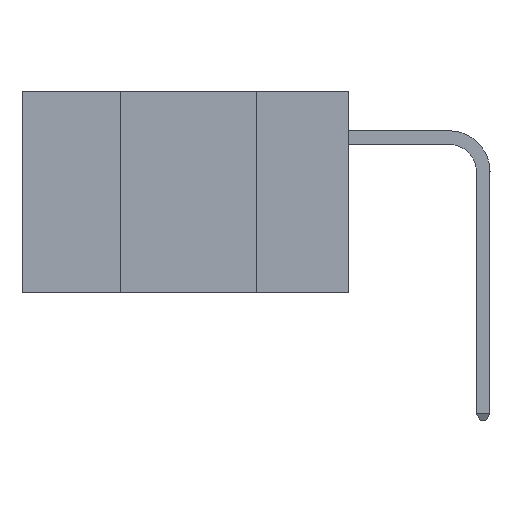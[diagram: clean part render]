
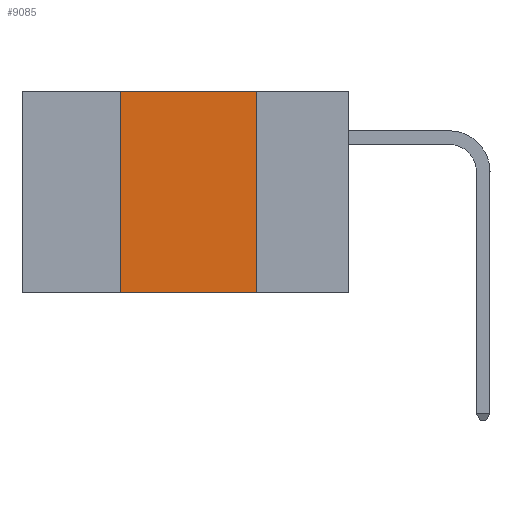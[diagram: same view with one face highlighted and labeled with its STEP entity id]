
A CAD part, left-side view. The second image highlights one B-rep face of the part: STEP entity #9085.
In plain terms, the highlighted planar face has unit normal (-1, 0, 0).
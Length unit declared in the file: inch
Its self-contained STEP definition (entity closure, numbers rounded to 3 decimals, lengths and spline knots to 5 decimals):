
#178 = EDGE_LOOP ( 'NONE', ( #279, #3613, #8611, #1136 ) ) ;
#191 = VERTEX_POINT ( 'NONE', #4057 ) ;
#196 = VERTEX_POINT ( 'NONE', #4852 ) ;
#248 = DIRECTION ( 'NONE',  ( 1., 0., 0. ) ) ;
#279 = ORIENTED_EDGE ( 'NONE', *, *, #11119, .F. ) ;
#324 = DIRECTION ( 'NONE',  ( 0., 0., -1. ) ) ;
#400 = VECTOR ( 'NONE', #6209, 39.37008 ) ;
#1136 = ORIENTED_EDGE ( 'NONE', *, *, #6292, .T. ) ;
#1655 = VERTEX_POINT ( 'NONE', #6660 ) ;
#2400 = CARTESIAN_POINT ( 'NONE',  ( 0., 0.42, 0. ) ) ;
#3613 = ORIENTED_EDGE ( 'NONE', *, *, #4867, .F. ) ;
#3620 = LINE ( 'NONE', #2400, #400 ) ;
#3752 = CARTESIAN_POINT ( 'NONE',  ( 0., 0.6, -0.37 ) ) ;
#4057 = CARTESIAN_POINT ( 'NONE',  ( 0., 0.17, 0. ) ) ;
#4496 = CARTESIAN_POINT ( 'NONE',  ( 0., 0.6, 0. ) ) ;
#4852 = CARTESIAN_POINT ( 'NONE',  ( 0., 0.42, 0. ) ) ;
#4867 = EDGE_CURVE ( 'NONE', #196, #191, #10210, .T. ) ;
#5749 = FACE_OUTER_BOUND ( 'NONE', #178, .T. ) ;
#6209 = DIRECTION ( 'NONE',  ( 0., 0., 1. ) ) ;
#6292 = EDGE_CURVE ( 'NONE', #9294, #1655, #9426, .T. ) ;
#6634 = LINE ( 'NONE', #7870, #11898 ) ;
#6660 = CARTESIAN_POINT ( 'NONE',  ( 0., 0.17, -0.37 ) ) ;
#7106 = VECTOR ( 'NONE', #9514, 39.37008 ) ;
#7370 = EDGE_CURVE ( 'NONE', #9294, #196, #3620, .T. ) ;
#7865 = VECTOR ( 'NONE', #10993, 39.37008 ) ;
#7870 = CARTESIAN_POINT ( 'NONE',  ( 0., 0.17, 0. ) ) ;
#8611 = ORIENTED_EDGE ( 'NONE', *, *, #7370, .F. ) ;
#8653 = CARTESIAN_POINT ( 'NONE',  ( 0., 0.6, 0. ) ) ;
#9085 = ADVANCED_FACE ( 'NONE', ( #5749 ), #11395, .F. ) ;
#9294 = VERTEX_POINT ( 'NONE', #10047 ) ;
#9426 = LINE ( 'NONE', #3752, #7106 ) ;
#9514 = DIRECTION ( 'NONE',  ( 0., -1., 0. ) ) ;
#9668 = AXIS2_PLACEMENT_3D ( 'NONE', #8653, #248, #324 ) ;
#9745 = DIRECTION ( 'NONE',  ( 0., 0., -1. ) ) ;
#10047 = CARTESIAN_POINT ( 'NONE',  ( 0., 0.42, -0.37 ) ) ;
#10210 = LINE ( 'NONE', #4496, #7865 ) ;
#10993 = DIRECTION ( 'NONE',  ( 0., -1., 0. ) ) ;
#11119 = EDGE_CURVE ( 'NONE', #191, #1655, #6634, .T. ) ;
#11395 = PLANE ( 'NONE',  #9668 ) ;
#11898 = VECTOR ( 'NONE', #9745, 39.37008 ) ;
